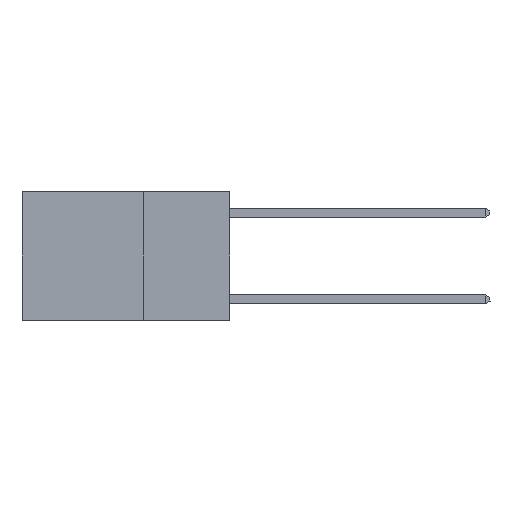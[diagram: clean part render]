
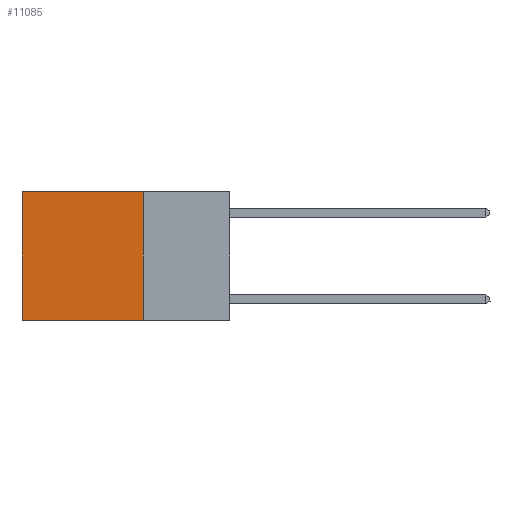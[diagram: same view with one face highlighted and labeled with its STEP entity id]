
A CAD part, left-side view. The second image highlights one B-rep face of the part: STEP entity #11085.
In plain terms, the highlighted planar face has unit normal (-1, 0, 0).
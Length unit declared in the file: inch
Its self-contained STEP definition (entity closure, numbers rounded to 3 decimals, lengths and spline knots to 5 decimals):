
#484 = CARTESIAN_POINT ( 'NONE',  ( 0.2625, 0.6, -0.37 ) ) ;
#695 = VECTOR ( 'NONE', #20304, 39.37008 ) ;
#1097 = ORIENTED_EDGE ( 'NONE', *, *, #20401, .F. ) ;
#2686 = CARTESIAN_POINT ( 'NONE',  ( 0.2625, 0.25, 0. ) ) ;
#3685 = VECTOR ( 'NONE', #13900, 39.37008 ) ;
#4400 = VERTEX_POINT ( 'NONE', #484 ) ;
#4800 = DIRECTION ( 'NONE',  ( 0., 0., -1. ) ) ;
#4907 = EDGE_CURVE ( 'NONE', #21808, #14143, #8388, .T. ) ;
#5165 = CARTESIAN_POINT ( 'NONE',  ( 0.2625, 0.25, 0. ) ) ;
#5488 = DIRECTION ( 'NONE',  ( 0., 0., -1. ) ) ;
#5604 = CARTESIAN_POINT ( 'NONE',  ( 0.2625, 0.6, 0. ) ) ;
#6174 = CARTESIAN_POINT ( 'NONE',  ( 0.2625, 0.25, -0.37 ) ) ;
#7325 = VERTEX_POINT ( 'NONE', #12925 ) ;
#7564 = EDGE_CURVE ( 'NONE', #7325, #4400, #18435, .T. ) ;
#8388 = LINE ( 'NONE', #5165, #3685 ) ;
#10699 = ORIENTED_EDGE ( 'NONE', *, *, #7564, .F. ) ;
#11085 = ADVANCED_FACE ( 'NONE', ( #19321 ), #20748, .F. ) ;
#11126 = EDGE_LOOP ( 'NONE', ( #17095, #10699, #1097, #16439 ) ) ;
#12925 = CARTESIAN_POINT ( 'NONE',  ( 0.2625, 0.25, -0.37 ) ) ;
#13608 = VECTOR ( 'NONE', #17779, 39.37008 ) ;
#13900 = DIRECTION ( 'NONE',  ( 0., 1., 0. ) ) ;
#14143 = VERTEX_POINT ( 'NONE', #5604 ) ;
#14157 = CARTESIAN_POINT ( 'NONE',  ( 0.2625, 0.6, 0. ) ) ;
#15006 = LINE ( 'NONE', #14157, #17520 ) ;
#15333 = AXIS2_PLACEMENT_3D ( 'NONE', #15527, #22932, #4800 ) ;
#15527 = CARTESIAN_POINT ( 'NONE',  ( 0.2625, 0.25, 0. ) ) ;
#15834 = CARTESIAN_POINT ( 'NONE',  ( 0.2625, 0.25, 0. ) ) ;
#16439 = ORIENTED_EDGE ( 'NONE', *, *, #4907, .T. ) ;
#17095 = ORIENTED_EDGE ( 'NONE', *, *, #20927, .T. ) ;
#17520 = VECTOR ( 'NONE', #5488, 39.37008 ) ;
#17779 = DIRECTION ( 'NONE',  ( 0., 0., -1. ) ) ;
#18435 = LINE ( 'NONE', #6174, #695 ) ;
#19321 = FACE_OUTER_BOUND ( 'NONE', #11126, .T. ) ;
#20304 = DIRECTION ( 'NONE',  ( 0., 1., 0. ) ) ;
#20401 = EDGE_CURVE ( 'NONE', #21808, #7325, #21289, .T. ) ;
#20748 = PLANE ( 'NONE',  #15333 ) ;
#20927 = EDGE_CURVE ( 'NONE', #14143, #4400, #15006, .T. ) ;
#21289 = LINE ( 'NONE', #15834, #13608 ) ;
#21808 = VERTEX_POINT ( 'NONE', #2686 ) ;
#22932 = DIRECTION ( 'NONE',  ( 1., 0., 0. ) ) ;
